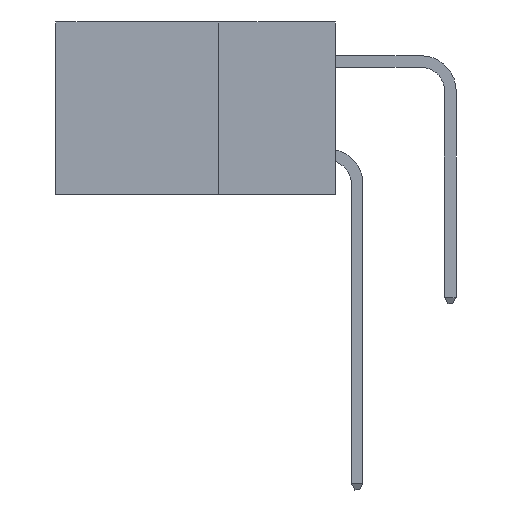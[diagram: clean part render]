
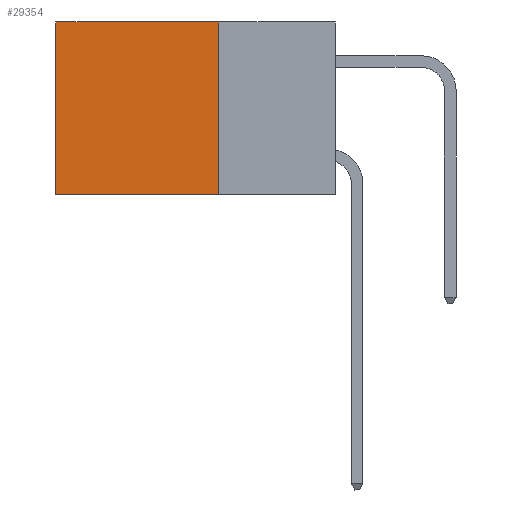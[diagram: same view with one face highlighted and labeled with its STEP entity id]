
A CAD part, left-side view. The second image highlights one B-rep face of the part: STEP entity #29354.
In plain terms, the highlighted planar face has unit normal (-1, 0, 0).
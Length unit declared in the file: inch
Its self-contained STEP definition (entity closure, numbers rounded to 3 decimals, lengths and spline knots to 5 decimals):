
#2201 = CARTESIAN_POINT ( 'NONE',  ( 0.2875, 0.25, 0. ) ) ;
#2897 = AXIS2_PLACEMENT_3D ( 'NONE', #43656, #23120, #19451 ) ;
#3539 = CARTESIAN_POINT ( 'NONE',  ( 0.2875, 0.25, -0.37 ) ) ;
#3810 = VECTOR ( 'NONE', #43351, 39.37008 ) ;
#5590 = EDGE_CURVE ( 'NONE', #15543, #26616, #30813, .T. ) ;
#5673 = VECTOR ( 'NONE', #16055, 39.37008 ) ;
#8942 = ORIENTED_EDGE ( 'NONE', *, *, #5590, .F. ) ;
#10667 = CARTESIAN_POINT ( 'NONE',  ( 0.2875, 0.25, 0. ) ) ;
#10883 = LINE ( 'NONE', #10667, #17743 ) ;
#12846 = CARTESIAN_POINT ( 'NONE',  ( 0.2875, 0.25, -0.37 ) ) ;
#15543 = VERTEX_POINT ( 'NONE', #2201 ) ;
#15845 = EDGE_CURVE ( 'NONE', #34594, #28232, #42912, .T. ) ;
#16055 = DIRECTION ( 'NONE',  ( 0., 1., 0. ) ) ;
#17323 = EDGE_CURVE ( 'NONE', #15543, #34594, #10883, .T. ) ;
#17743 = VECTOR ( 'NONE', #35954, 39.37008 ) ;
#18791 = VECTOR ( 'NONE', #26434, 39.37008 ) ;
#18992 = PLANE ( 'NONE',  #2897 ) ;
#19451 = DIRECTION ( 'NONE',  ( 0., 0., -1. ) ) ;
#22374 = CARTESIAN_POINT ( 'NONE',  ( 0.2875, 0.6, 0. ) ) ;
#23120 = DIRECTION ( 'NONE',  ( 1., 0., 0. ) ) ;
#23789 = EDGE_LOOP ( 'NONE', ( #33805, #31427, #8942, #43166 ) ) ;
#26398 = LINE ( 'NONE', #12846, #5673 ) ;
#26434 = DIRECTION ( 'NONE',  ( 0., 0., -1. ) ) ;
#26616 = VERTEX_POINT ( 'NONE', #3539 ) ;
#28232 = VERTEX_POINT ( 'NONE', #44075 ) ;
#29354 = ADVANCED_FACE ( 'NONE', ( #40888 ), #18992, .F. ) ;
#30813 = LINE ( 'NONE', #37052, #18791 ) ;
#31427 = ORIENTED_EDGE ( 'NONE', *, *, #39564, .F. ) ;
#32853 = CARTESIAN_POINT ( 'NONE',  ( 0.2875, 0.6, 0. ) ) ;
#33805 = ORIENTED_EDGE ( 'NONE', *, *, #15845, .T. ) ;
#34594 = VERTEX_POINT ( 'NONE', #32853 ) ;
#35954 = DIRECTION ( 'NONE',  ( 0., 1., 0. ) ) ;
#37052 = CARTESIAN_POINT ( 'NONE',  ( 0.2875, 0.25, 0. ) ) ;
#39564 = EDGE_CURVE ( 'NONE', #26616, #28232, #26398, .T. ) ;
#40888 = FACE_OUTER_BOUND ( 'NONE', #23789, .T. ) ;
#42912 = LINE ( 'NONE', #22374, #3810 ) ;
#43166 = ORIENTED_EDGE ( 'NONE', *, *, #17323, .T. ) ;
#43351 = DIRECTION ( 'NONE',  ( 0., 0., -1. ) ) ;
#43656 = CARTESIAN_POINT ( 'NONE',  ( 0.2875, 0.25, 0. ) ) ;
#44075 = CARTESIAN_POINT ( 'NONE',  ( 0.2875, 0.6, -0.37 ) ) ;
